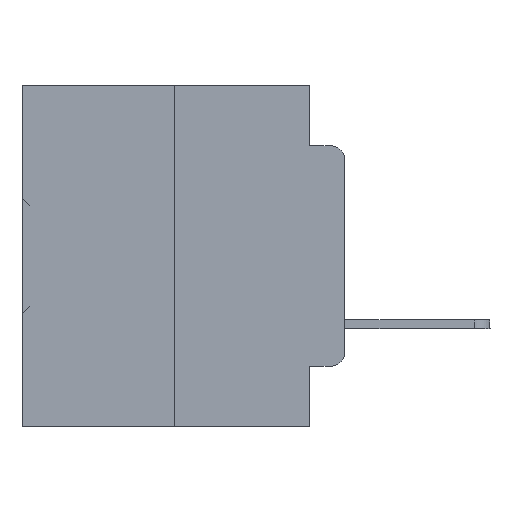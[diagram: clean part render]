
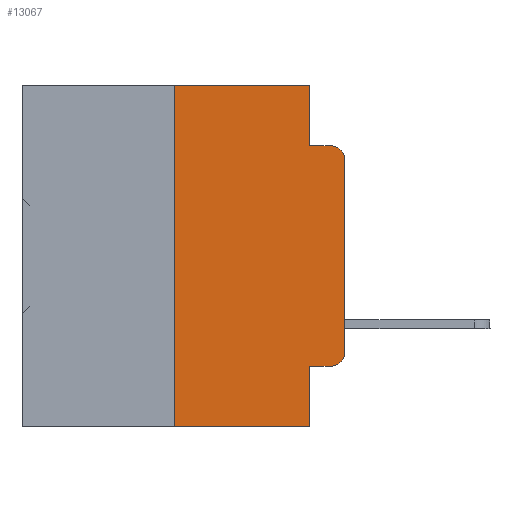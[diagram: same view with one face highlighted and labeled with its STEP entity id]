
A CAD part, left-side view. The second image highlights one B-rep face of the part: STEP entity #13067.
In plain terms, the highlighted planar face has unit normal (-1, 0, 0).
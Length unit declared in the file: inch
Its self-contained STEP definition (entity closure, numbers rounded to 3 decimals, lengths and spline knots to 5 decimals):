
#406 = CARTESIAN_POINT ( 'NONE',  ( 0., 0.051, -0.0885 ) ) ;
#578 = DIRECTION ( 'NONE',  ( 0., 0., -1. ) ) ;
#913 = CARTESIAN_POINT ( 'NONE',  ( 0., 0.051, -0.5 ) ) ;
#954 = VECTOR ( 'NONE', #13560, 39.37008 ) ;
#1346 = CARTESIAN_POINT ( 'NONE',  ( 0., 0., -0.3915 ) ) ;
#2291 = ORIENTED_EDGE ( 'NONE', *, *, #22937, .T. ) ;
#2532 = VECTOR ( 'NONE', #14648, 39.37008 ) ;
#3205 = AXIS2_PLACEMENT_3D ( 'NONE', #22022, #14056, #19793 ) ;
#3360 = VECTOR ( 'NONE', #19822, 39.37008 ) ;
#3386 = EDGE_CURVE ( 'NONE', #29155, #34941, #26902, .T. ) ;
#4788 = EDGE_CURVE ( 'NONE', #29155, #12249, #18859, .T. ) ;
#4861 = EDGE_LOOP ( 'NONE', ( #35229, #6922, #12824, #5252, #8496, #8598, #20003, #12483, #6210, #2291 ) ) ;
#5252 = ORIENTED_EDGE ( 'NONE', *, *, #21616, .F. ) ;
#5619 = CIRCLE ( 'NONE', #7758, 0.02 ) ;
#6210 = ORIENTED_EDGE ( 'NONE', *, *, #3386, .T. ) ;
#6597 = VERTEX_POINT ( 'NONE', #1346 ) ;
#6601 = CARTESIAN_POINT ( 'NONE',  ( 0., 0.25, -0.5 ) ) ;
#6922 = ORIENTED_EDGE ( 'NONE', *, *, #23540, .T. ) ;
#6933 = CARTESIAN_POINT ( 'NONE',  ( 0., 0., -0.1085 ) ) ;
#7106 = VERTEX_POINT ( 'NONE', #14355 ) ;
#7223 = CARTESIAN_POINT ( 'NONE',  ( 0., 0.02, -0.1085 ) ) ;
#7333 = DIRECTION ( 'NONE',  ( 0., 0., -1. ) ) ;
#7758 = AXIS2_PLACEMENT_3D ( 'NONE', #7223, #21717, #27420 ) ;
#7995 = VECTOR ( 'NONE', #25931, 39.37008 ) ;
#8496 = ORIENTED_EDGE ( 'NONE', *, *, #28311, .F. ) ;
#8598 = ORIENTED_EDGE ( 'NONE', *, *, #28393, .F. ) ;
#9319 = VECTOR ( 'NONE', #10032, 39.37008 ) ;
#9615 = CARTESIAN_POINT ( 'NONE',  ( 0., 0.02, -0.4115 ) ) ;
#10032 = DIRECTION ( 'NONE',  ( 0., 0., -1. ) ) ;
#10429 = CARTESIAN_POINT ( 'NONE',  ( 0., 0.02, -0.3915 ) ) ;
#11019 = LINE ( 'NONE', #24932, #11844 ) ;
#11179 = LINE ( 'NONE', #16646, #954 ) ;
#11800 = CARTESIAN_POINT ( 'NONE',  ( 0., 0., 0. ) ) ;
#11844 = VECTOR ( 'NONE', #25049, 39.37008 ) ;
#12249 = VERTEX_POINT ( 'NONE', #913 ) ;
#12483 = ORIENTED_EDGE ( 'NONE', *, *, #4788, .F. ) ;
#12824 = ORIENTED_EDGE ( 'NONE', *, *, #31085, .F. ) ;
#13067 = ADVANCED_FACE ( 'NONE', ( #28489 ), #21148, .F. ) ;
#13560 = DIRECTION ( 'NONE',  ( 0., 0., 1. ) ) ;
#14056 = DIRECTION ( 'NONE',  ( 1., 0., 0. ) ) ;
#14105 = VECTOR ( 'NONE', #31331, 39.37008 ) ;
#14355 = CARTESIAN_POINT ( 'NONE',  ( 0., 0.02, -0.0885 ) ) ;
#14461 = CARTESIAN_POINT ( 'NONE',  ( 0., 0.473, 0. ) ) ;
#14578 = CARTESIAN_POINT ( 'NONE',  ( 0., 0.051, 0. ) ) ;
#14648 = DIRECTION ( 'NONE',  ( 0., 0., 1. ) ) ;
#16173 = EDGE_CURVE ( 'NONE', #31340, #12249, #11019, .T. ) ;
#16646 = CARTESIAN_POINT ( 'NONE',  ( 0., 0.25, 0. ) ) ;
#17052 = CARTESIAN_POINT ( 'NONE',  ( 0., 0.051, 0. ) ) ;
#18859 = LINE ( 'NONE', #14578, #26805 ) ;
#19164 = LINE ( 'NONE', #21807, #9319 ) ;
#19360 = EDGE_CURVE ( 'NONE', #6597, #27554, #25083, .T. ) ;
#19480 = CIRCLE ( 'NONE', #24840, 0.02 ) ;
#19562 = LINE ( 'NONE', #34388, #7995 ) ;
#19700 = VERTEX_POINT ( 'NONE', #17052 ) ;
#19793 = DIRECTION ( 'NONE',  ( 0., 0., -1. ) ) ;
#19822 = DIRECTION ( 'NONE',  ( 0., -1., 0. ) ) ;
#20003 = ORIENTED_EDGE ( 'NONE', *, *, #16173, .T. ) ;
#21148 = PLANE ( 'NONE',  #3205 ) ;
#21616 = EDGE_CURVE ( 'NONE', #19700, #33840, #19164, .T. ) ;
#21717 = DIRECTION ( 'NONE',  ( -1., 0., 0. ) ) ;
#21807 = CARTESIAN_POINT ( 'NONE',  ( 0., 0.051, 0. ) ) ;
#22022 = CARTESIAN_POINT ( 'NONE',  ( 0., 0.473, 0. ) ) ;
#22937 = EDGE_CURVE ( 'NONE', #34941, #6597, #19480, .T. ) ;
#23540 = EDGE_CURVE ( 'NONE', #27554, #7106, #5619, .T. ) ;
#24342 = LINE ( 'NONE', #14461, #14105 ) ;
#24840 = AXIS2_PLACEMENT_3D ( 'NONE', #10429, #35589, #7333 ) ;
#24932 = CARTESIAN_POINT ( 'NONE',  ( 0., 0.473, -0.5 ) ) ;
#25022 = CARTESIAN_POINT ( 'NONE',  ( 0., 0.051, -0.4115 ) ) ;
#25049 = DIRECTION ( 'NONE',  ( 0., -1., 0. ) ) ;
#25083 = LINE ( 'NONE', #11800, #2532 ) ;
#25931 = DIRECTION ( 'NONE',  ( 0., -1., 0. ) ) ;
#26805 = VECTOR ( 'NONE', #578, 39.37008 ) ;
#26902 = LINE ( 'NONE', #25022, #3360 ) ;
#27420 = DIRECTION ( 'NONE',  ( 0., 0., -1. ) ) ;
#27554 = VERTEX_POINT ( 'NONE', #6933 ) ;
#28311 = EDGE_CURVE ( 'NONE', #35289, #19700, #24342, .T. ) ;
#28393 = EDGE_CURVE ( 'NONE', #31340, #35289, #11179, .T. ) ;
#28489 = FACE_OUTER_BOUND ( 'NONE', #4861, .T. ) ;
#29155 = VERTEX_POINT ( 'NONE', #34900 ) ;
#31085 = EDGE_CURVE ( 'NONE', #33840, #7106, #19562, .T. ) ;
#31331 = DIRECTION ( 'NONE',  ( 0., -1., 0. ) ) ;
#31340 = VERTEX_POINT ( 'NONE', #6601 ) ;
#31961 = CARTESIAN_POINT ( 'NONE',  ( 0., 0.25, 0. ) ) ;
#33840 = VERTEX_POINT ( 'NONE', #406 ) ;
#34388 = CARTESIAN_POINT ( 'NONE',  ( 0., 0.051, -0.0885 ) ) ;
#34900 = CARTESIAN_POINT ( 'NONE',  ( 0., 0.051, -0.4115 ) ) ;
#34941 = VERTEX_POINT ( 'NONE', #9615 ) ;
#35229 = ORIENTED_EDGE ( 'NONE', *, *, #19360, .T. ) ;
#35289 = VERTEX_POINT ( 'NONE', #31961 ) ;
#35589 = DIRECTION ( 'NONE',  ( -1., 0., 0. ) ) ;
